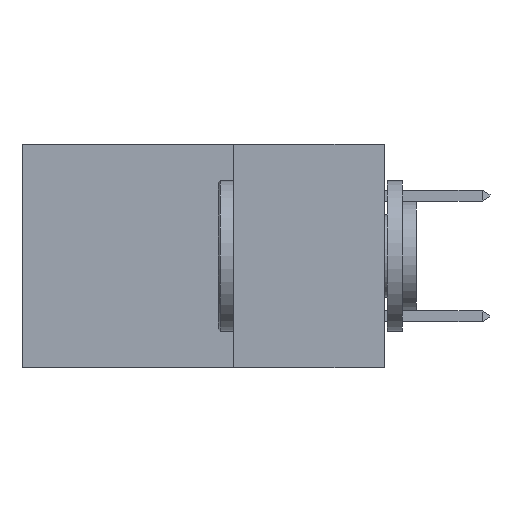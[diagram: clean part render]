
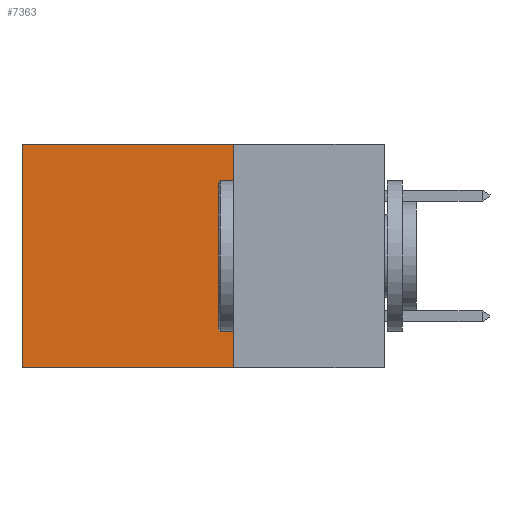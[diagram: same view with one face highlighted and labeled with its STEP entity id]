
A CAD part, left-side view. The second image highlights one B-rep face of the part: STEP entity #7363.
In plain terms, the highlighted planar face has unit normal (-1, 0, 0).
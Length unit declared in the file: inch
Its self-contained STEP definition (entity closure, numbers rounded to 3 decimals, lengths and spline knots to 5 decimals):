
#90 = CARTESIAN_POINT ( 'NONE',  ( 0.2875, 0.25, 0. ) ) ;
#875 = LINE ( 'NONE', #6164, #5073 ) ;
#1708 = LINE ( 'NONE', #6295, #5059 ) ;
#1973 = VERTEX_POINT ( 'NONE', #90 ) ;
#2141 = DIRECTION ( 'NONE',  ( 0., 0., -1. ) ) ;
#2187 = ORIENTED_EDGE ( 'NONE', *, *, #8909, .T. ) ;
#2370 = VECTOR ( 'NONE', #8821, 39.37008 ) ;
#2689 = DIRECTION ( 'NONE',  ( 0., 1., 0. ) ) ;
#2731 = VERTEX_POINT ( 'NONE', #3013 ) ;
#2949 = CARTESIAN_POINT ( 'NONE',  ( 0.2875, 0.25, -0.37 ) ) ;
#3013 = CARTESIAN_POINT ( 'NONE',  ( 0.2875, 0.6, 0. ) ) ;
#3232 = FACE_OUTER_BOUND ( 'NONE', #6092, .T. ) ;
#3585 = VERTEX_POINT ( 'NONE', #2949 ) ;
#3614 = DIRECTION ( 'NONE',  ( 0., 0., -1. ) ) ;
#4075 = CARTESIAN_POINT ( 'NONE',  ( 0.2875, 0.25, 0. ) ) ;
#4125 = CARTESIAN_POINT ( 'NONE',  ( 0.2875, 0.25, -0.37 ) ) ;
#5059 = VECTOR ( 'NONE', #2689, 39.37008 ) ;
#5073 = VECTOR ( 'NONE', #9763, 39.37008 ) ;
#5507 = ORIENTED_EDGE ( 'NONE', *, *, #7803, .F. ) ;
#6092 = EDGE_LOOP ( 'NONE', ( #2187, #10170, #5507, #8095 ) ) ;
#6164 = CARTESIAN_POINT ( 'NONE',  ( 0.2875, 0.25, 0. ) ) ;
#6295 = CARTESIAN_POINT ( 'NONE',  ( 0.2875, 0.25, 0. ) ) ;
#6430 = LINE ( 'NONE', #4125, #2370 ) ;
#7021 = VERTEX_POINT ( 'NONE', #9250 ) ;
#7188 = EDGE_CURVE ( 'NONE', #1973, #2731, #1708, .T. ) ;
#7363 = ADVANCED_FACE ( 'NONE', ( #3232 ), #7526, .F. ) ;
#7526 = PLANE ( 'NONE',  #10839 ) ;
#7803 = EDGE_CURVE ( 'NONE', #1973, #3585, #875, .T. ) ;
#8095 = ORIENTED_EDGE ( 'NONE', *, *, #7188, .T. ) ;
#8447 = VECTOR ( 'NONE', #3614, 39.37008 ) ;
#8821 = DIRECTION ( 'NONE',  ( 0., 1., 0. ) ) ;
#8909 = EDGE_CURVE ( 'NONE', #2731, #7021, #9701, .T. ) ;
#9026 = CARTESIAN_POINT ( 'NONE',  ( 0.2875, 0.6, 0. ) ) ;
#9250 = CARTESIAN_POINT ( 'NONE',  ( 0.2875, 0.6, -0.37 ) ) ;
#9361 = EDGE_CURVE ( 'NONE', #3585, #7021, #6430, .T. ) ;
#9701 = LINE ( 'NONE', #9026, #8447 ) ;
#9763 = DIRECTION ( 'NONE',  ( 0., 0., -1. ) ) ;
#10170 = ORIENTED_EDGE ( 'NONE', *, *, #9361, .F. ) ;
#10357 = DIRECTION ( 'NONE',  ( 1., 0., 0. ) ) ;
#10839 = AXIS2_PLACEMENT_3D ( 'NONE', #4075, #10357, #2141 ) ;
